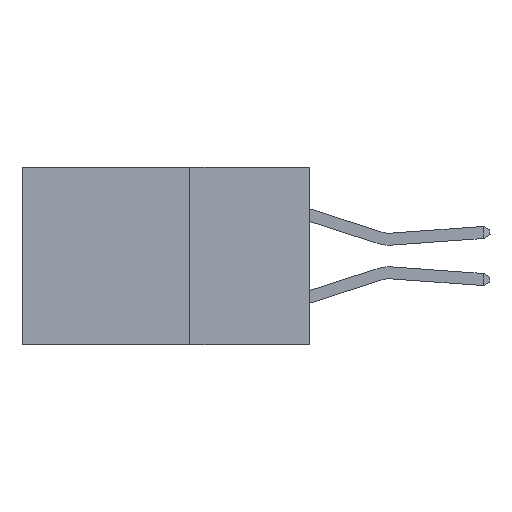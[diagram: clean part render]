
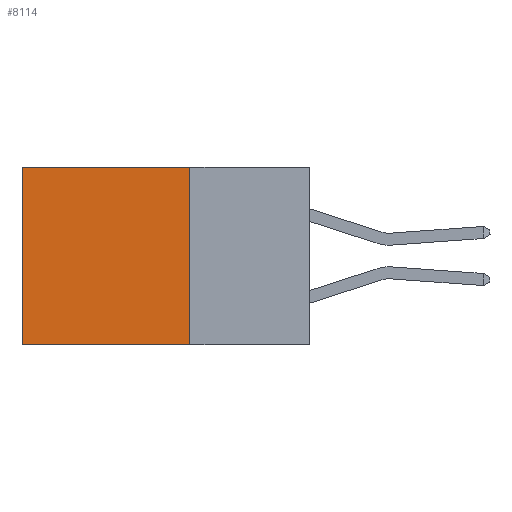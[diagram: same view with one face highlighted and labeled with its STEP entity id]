
A CAD part, left-side view. The second image highlights one B-rep face of the part: STEP entity #8114.
In plain terms, the highlighted planar face has unit normal (-1, 0, 0).
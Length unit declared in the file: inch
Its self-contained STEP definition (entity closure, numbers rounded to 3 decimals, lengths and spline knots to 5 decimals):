
#71 = AXIS2_PLACEMENT_3D ( 'NONE', #7579, #8259, #2437 ) ;
#75 = DIRECTION ( 'NONE',  ( 0., 0., -1. ) ) ;
#728 = ORIENTED_EDGE ( 'NONE', *, *, #9295, .F. ) ;
#1321 = VECTOR ( 'NONE', #5817, 39.37008 ) ;
#1767 = EDGE_CURVE ( 'NONE', #5125, #2126, #3389, .T. ) ;
#2059 = CARTESIAN_POINT ( 'NONE',  ( 0.298, 0.25, 0. ) ) ;
#2126 = VERTEX_POINT ( 'NONE', #7797 ) ;
#2240 = CARTESIAN_POINT ( 'NONE',  ( 0.298, 0.25, -0.37 ) ) ;
#2423 = LINE ( 'NONE', #4403, #3319 ) ;
#2437 = DIRECTION ( 'NONE',  ( 0., 0., -1. ) ) ;
#3006 = DIRECTION ( 'NONE',  ( 0., 0., -1. ) ) ;
#3017 = ORIENTED_EDGE ( 'NONE', *, *, #1767, .T. ) ;
#3319 = VECTOR ( 'NONE', #3006, 39.37008 ) ;
#3389 = LINE ( 'NONE', #9278, #5076 ) ;
#3406 = ORIENTED_EDGE ( 'NONE', *, *, #5403, .T. ) ;
#3521 = DIRECTION ( 'NONE',  ( 0., 1., 0. ) ) ;
#3912 = LINE ( 'NONE', #8755, #8419 ) ;
#4012 = VERTEX_POINT ( 'NONE', #6091 ) ;
#4403 = CARTESIAN_POINT ( 'NONE',  ( 0.298, 0.6, 0. ) ) ;
#4694 = FACE_OUTER_BOUND ( 'NONE', #9247, .T. ) ;
#5063 = CARTESIAN_POINT ( 'NONE',  ( 0.298, 0.25, -0.37 ) ) ;
#5076 = VECTOR ( 'NONE', #3521, 39.37008 ) ;
#5125 = VERTEX_POINT ( 'NONE', #2059 ) ;
#5336 = ORIENTED_EDGE ( 'NONE', *, *, #7613, .F. ) ;
#5372 = VERTEX_POINT ( 'NONE', #2240 ) ;
#5403 = EDGE_CURVE ( 'NONE', #2126, #4012, #2423, .T. ) ;
#5817 = DIRECTION ( 'NONE',  ( 0., 1., 0. ) ) ;
#6091 = CARTESIAN_POINT ( 'NONE',  ( 0.298, 0.6, -0.37 ) ) ;
#6430 = LINE ( 'NONE', #5063, #1321 ) ;
#6806 = PLANE ( 'NONE',  #71 ) ;
#7579 = CARTESIAN_POINT ( 'NONE',  ( 0.298, 0.25, 0. ) ) ;
#7613 = EDGE_CURVE ( 'NONE', #5372, #4012, #6430, .T. ) ;
#7797 = CARTESIAN_POINT ( 'NONE',  ( 0.298, 0.6, 0. ) ) ;
#8114 = ADVANCED_FACE ( 'NONE', ( #4694 ), #6806, .F. ) ;
#8259 = DIRECTION ( 'NONE',  ( 1., 0., 0. ) ) ;
#8419 = VECTOR ( 'NONE', #75, 39.37008 ) ;
#8755 = CARTESIAN_POINT ( 'NONE',  ( 0.298, 0.25, 0. ) ) ;
#9247 = EDGE_LOOP ( 'NONE', ( #3406, #5336, #728, #3017 ) ) ;
#9278 = CARTESIAN_POINT ( 'NONE',  ( 0.298, 0.25, 0. ) ) ;
#9295 = EDGE_CURVE ( 'NONE', #5125, #5372, #3912, .T. ) ;
